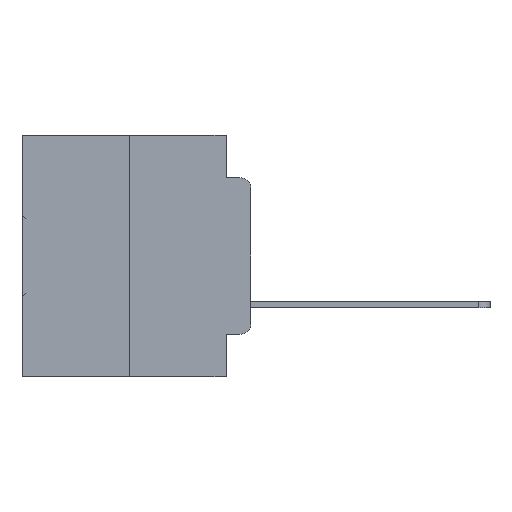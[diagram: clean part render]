
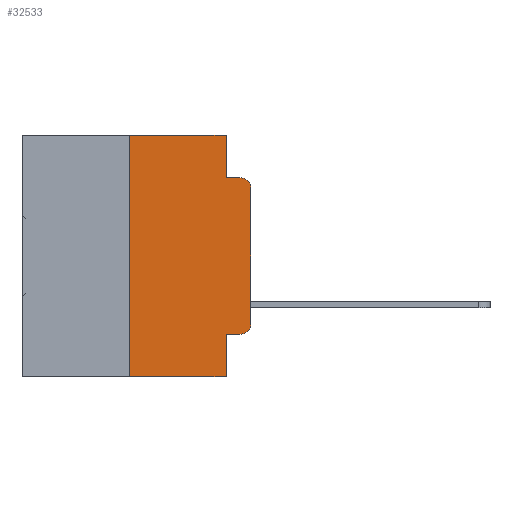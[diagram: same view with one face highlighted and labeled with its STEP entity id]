
A CAD part, left-side view. The second image highlights one B-rep face of the part: STEP entity #32533.
In plain terms, the highlighted planar face has unit normal (-1, 0, 0).
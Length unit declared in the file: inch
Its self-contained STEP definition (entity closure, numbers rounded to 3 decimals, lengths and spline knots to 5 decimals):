
#105 = VECTOR ( 'NONE', #15145, 39.37008 ) ;
#402 = VERTEX_POINT ( 'NONE', #10509 ) ;
#522 = CARTESIAN_POINT ( 'NONE',  ( 0., 0.051, -0.4115 ) ) ;
#1463 = VERTEX_POINT ( 'NONE', #16718 ) ;
#1586 = CARTESIAN_POINT ( 'NONE',  ( 0., 0.051, 0. ) ) ;
#1605 = DIRECTION ( 'NONE',  ( 0., -1., 0. ) ) ;
#1719 = CARTESIAN_POINT ( 'NONE',  ( 0., 0.051, -0.4115 ) ) ;
#2416 = VERTEX_POINT ( 'NONE', #522 ) ;
#2546 = CARTESIAN_POINT ( 'NONE',  ( 0., 0.25, -0.5 ) ) ;
#2772 = ORIENTED_EDGE ( 'NONE', *, *, #17347, .T. ) ;
#3595 = DIRECTION ( 'NONE',  ( -1., 0., 0. ) ) ;
#3642 = CARTESIAN_POINT ( 'NONE',  ( 0., 0.473, 0. ) ) ;
#3759 = VECTOR ( 'NONE', #27454, 39.37008 ) ;
#4477 = ORIENTED_EDGE ( 'NONE', *, *, #18251, .T. ) ;
#4933 = VECTOR ( 'NONE', #16655, 39.37008 ) ;
#5004 = ORIENTED_EDGE ( 'NONE', *, *, #18339, .F. ) ;
#6285 = LINE ( 'NONE', #24832, #20431 ) ;
#6340 = DIRECTION ( 'NONE',  ( 0., 0., -1. ) ) ;
#7898 = CARTESIAN_POINT ( 'NONE',  ( 0., 0.02, -0.3915 ) ) ;
#8161 = VERTEX_POINT ( 'NONE', #32170 ) ;
#9064 = CARTESIAN_POINT ( 'NONE',  ( 0., 0.473, 0. ) ) ;
#9278 = LINE ( 'NONE', #1586, #15424 ) ;
#9285 = DIRECTION ( 'NONE',  ( 0., -1., 0. ) ) ;
#9451 = VERTEX_POINT ( 'NONE', #17429 ) ;
#10188 = VERTEX_POINT ( 'NONE', #16649 ) ;
#10509 = CARTESIAN_POINT ( 'NONE',  ( 0., 0.02, -0.4115 ) ) ;
#10575 = DIRECTION ( 'NONE',  ( 0., 0., -1. ) ) ;
#11285 = VERTEX_POINT ( 'NONE', #32057 ) ;
#13417 = LINE ( 'NONE', #31977, #24710 ) ;
#13514 = AXIS2_PLACEMENT_3D ( 'NONE', #3642, #22188, #6340 ) ;
#14022 = CARTESIAN_POINT ( 'NONE',  ( 0., 0., 0. ) ) ;
#14516 = AXIS2_PLACEMENT_3D ( 'NONE', #7898, #25993, #10575 ) ;
#14631 = ORIENTED_EDGE ( 'NONE', *, *, #18298, .F. ) ;
#15145 = DIRECTION ( 'NONE',  ( 0., -1., 0. ) ) ;
#15424 = VECTOR ( 'NONE', #27658, 39.37008 ) ;
#15601 = FACE_OUTER_BOUND ( 'NONE', #19129, .T. ) ;
#15602 = EDGE_CURVE ( 'NONE', #20053, #25985, #27828, .T. ) ;
#16649 = CARTESIAN_POINT ( 'NONE',  ( 0., 0.02, -0.0885 ) ) ;
#16655 = DIRECTION ( 'NONE',  ( 0., 0., 1. ) ) ;
#16718 = CARTESIAN_POINT ( 'NONE',  ( 0., 0., -0.3915 ) ) ;
#16917 = AXIS2_PLACEMENT_3D ( 'NONE', #19532, #3595, #22149 ) ;
#17347 = EDGE_CURVE ( 'NONE', #18994, #11285, #18738, .T. ) ;
#17429 = CARTESIAN_POINT ( 'NONE',  ( 0., 0.051, -0.0885 ) ) ;
#18205 = EDGE_CURVE ( 'NONE', #1463, #8161, #19071, .T. ) ;
#18251 = EDGE_CURVE ( 'NONE', #8161, #10188, #18262, .T. ) ;
#18262 = CIRCLE ( 'NONE', #16917, 0.02 ) ;
#18298 = EDGE_CURVE ( 'NONE', #9451, #10188, #6285, .T. ) ;
#18339 = EDGE_CURVE ( 'NONE', #25985, #9451, #13417, .T. ) ;
#18350 = EDGE_CURVE ( 'NONE', #18994, #20053, #30976, .T. ) ;
#18403 = EDGE_CURVE ( 'NONE', #2416, #11285, #9278, .T. ) ;
#18423 = CARTESIAN_POINT ( 'NONE',  ( 0., 0.051, 0. ) ) ;
#18442 = EDGE_CURVE ( 'NONE', #2416, #402, #21624, .T. ) ;
#18449 = EDGE_CURVE ( 'NONE', #402, #1463, #22393, .T. ) ;
#18628 = ORIENTED_EDGE ( 'NONE', *, *, #18350, .F. ) ;
#18738 = LINE ( 'NONE', #27673, #23963 ) ;
#18994 = VERTEX_POINT ( 'NONE', #2546 ) ;
#19071 = LINE ( 'NONE', #14022, #4933 ) ;
#19129 = EDGE_LOOP ( 'NONE', ( #24625, #4477, #14631, #5004, #29079, #18628, #2772, #29418, #30604, #31310 ) ) ;
#19532 = CARTESIAN_POINT ( 'NONE',  ( 0., 0.02, -0.1085 ) ) ;
#19883 = DIRECTION ( 'NONE',  ( 0., 0., -1. ) ) ;
#20053 = VERTEX_POINT ( 'NONE', #32453 ) ;
#20431 = VECTOR ( 'NONE', #9285, 39.37008 ) ;
#21351 = VECTOR ( 'NONE', #27040, 39.37008 ) ;
#21624 = LINE ( 'NONE', #1719, #105 ) ;
#22149 = DIRECTION ( 'NONE',  ( 0., 0., -1. ) ) ;
#22188 = DIRECTION ( 'NONE',  ( 1., 0., 0. ) ) ;
#22393 = CIRCLE ( 'NONE', #14516, 0.02 ) ;
#23963 = VECTOR ( 'NONE', #1605, 39.37008 ) ;
#24625 = ORIENTED_EDGE ( 'NONE', *, *, #18205, .T. ) ;
#24710 = VECTOR ( 'NONE', #19883, 39.37008 ) ;
#24832 = CARTESIAN_POINT ( 'NONE',  ( 0., 0.051, -0.0885 ) ) ;
#25035 = CARTESIAN_POINT ( 'NONE',  ( 0., 0.25, 0. ) ) ;
#25985 = VERTEX_POINT ( 'NONE', #18423 ) ;
#25993 = DIRECTION ( 'NONE',  ( -1., 0., 0. ) ) ;
#27040 = DIRECTION ( 'NONE',  ( 0., -1., 0. ) ) ;
#27454 = DIRECTION ( 'NONE',  ( 0., 0., 1. ) ) ;
#27658 = DIRECTION ( 'NONE',  ( 0., 0., -1. ) ) ;
#27673 = CARTESIAN_POINT ( 'NONE',  ( 0., 0.473, -0.5 ) ) ;
#27828 = LINE ( 'NONE', #9064, #21351 ) ;
#29079 = ORIENTED_EDGE ( 'NONE', *, *, #15602, .F. ) ;
#29418 = ORIENTED_EDGE ( 'NONE', *, *, #18403, .F. ) ;
#30604 = ORIENTED_EDGE ( 'NONE', *, *, #18442, .T. ) ;
#30976 = LINE ( 'NONE', #25035, #3759 ) ;
#31310 = ORIENTED_EDGE ( 'NONE', *, *, #18449, .T. ) ;
#31634 = PLANE ( 'NONE',  #13514 ) ;
#31977 = CARTESIAN_POINT ( 'NONE',  ( 0., 0.051, 0. ) ) ;
#32057 = CARTESIAN_POINT ( 'NONE',  ( 0., 0.051, -0.5 ) ) ;
#32170 = CARTESIAN_POINT ( 'NONE',  ( 0., 0., -0.1085 ) ) ;
#32453 = CARTESIAN_POINT ( 'NONE',  ( 0., 0.25, 0. ) ) ;
#32533 = ADVANCED_FACE ( 'NONE', ( #15601 ), #31634, .F. ) ;
